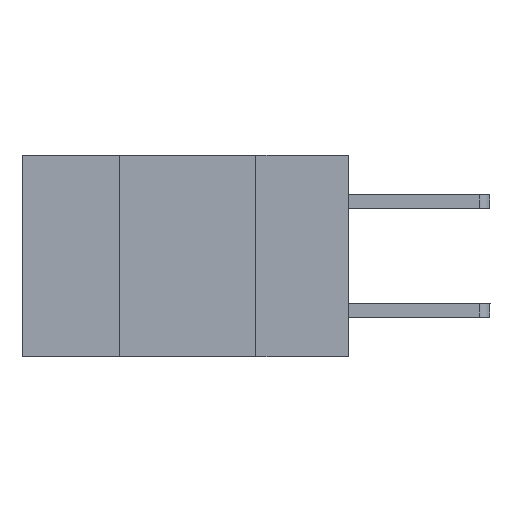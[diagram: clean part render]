
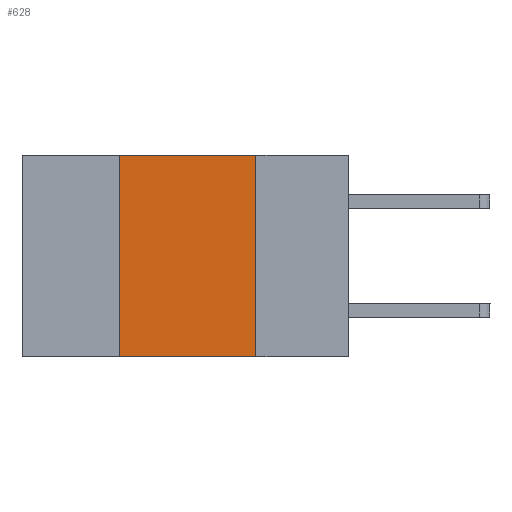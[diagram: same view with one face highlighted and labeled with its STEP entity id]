
A CAD part, left-side view. The second image highlights one B-rep face of the part: STEP entity #628.
In plain terms, the highlighted planar face has unit normal (-1, 0, 0).
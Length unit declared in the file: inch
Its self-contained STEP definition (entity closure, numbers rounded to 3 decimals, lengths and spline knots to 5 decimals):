
#43 = VECTOR ( 'NONE', #7409, 39.37008 ) ;
#469 = CARTESIAN_POINT ( 'NONE',  ( 0., 0.6, -0.37 ) ) ;
#628 = ADVANCED_FACE ( 'NONE', ( #2798 ), #4369, .F. ) ;
#1009 = CARTESIAN_POINT ( 'NONE',  ( 0., 0.17, 0. ) ) ;
#1123 = EDGE_CURVE ( 'NONE', #7954, #1808, #10056, .T. ) ;
#1143 = VECTOR ( 'NONE', #1589, 39.37008 ) ;
#1338 = LINE ( 'NONE', #1009, #43 ) ;
#1589 = DIRECTION ( 'NONE',  ( 0., 0., 1. ) ) ;
#1766 = EDGE_CURVE ( 'NONE', #7954, #2212, #9905, .T. ) ;
#1808 = VERTEX_POINT ( 'NONE', #9048 ) ;
#2044 = LINE ( 'NONE', #10238, #9132 ) ;
#2212 = VERTEX_POINT ( 'NONE', #3645 ) ;
#2516 = VERTEX_POINT ( 'NONE', #5108 ) ;
#2798 = FACE_OUTER_BOUND ( 'NONE', #9317, .T. ) ;
#2799 = DIRECTION ( 'NONE',  ( 1., 0., 0. ) ) ;
#3293 = ORIENTED_EDGE ( 'NONE', *, *, #1766, .F. ) ;
#3633 = DIRECTION ( 'NONE',  ( 0., -1., 0. ) ) ;
#3645 = CARTESIAN_POINT ( 'NONE',  ( 0., 0.42, 0. ) ) ;
#4081 = ORIENTED_EDGE ( 'NONE', *, *, #5012, .F. ) ;
#4369 = PLANE ( 'NONE',  #6369 ) ;
#5012 = EDGE_CURVE ( 'NONE', #2212, #2516, #2044, .T. ) ;
#5108 = CARTESIAN_POINT ( 'NONE',  ( 0., 0.17, 0. ) ) ;
#5318 = CARTESIAN_POINT ( 'NONE',  ( 0., 0.6, 0. ) ) ;
#5828 = ORIENTED_EDGE ( 'NONE', *, *, #8159, .F. ) ;
#5931 = ORIENTED_EDGE ( 'NONE', *, *, #1123, .T. ) ;
#6369 = AXIS2_PLACEMENT_3D ( 'NONE', #5318, #2799, #10193 ) ;
#6488 = CARTESIAN_POINT ( 'NONE',  ( 0., 0.42, 0. ) ) ;
#7409 = DIRECTION ( 'NONE',  ( 0., 0., -1. ) ) ;
#7812 = VECTOR ( 'NONE', #3633, 39.37008 ) ;
#7954 = VERTEX_POINT ( 'NONE', #10414 ) ;
#8159 = EDGE_CURVE ( 'NONE', #2516, #1808, #1338, .T. ) ;
#9048 = CARTESIAN_POINT ( 'NONE',  ( 0., 0.17, -0.37 ) ) ;
#9132 = VECTOR ( 'NONE', #9478, 39.37008 ) ;
#9317 = EDGE_LOOP ( 'NONE', ( #5828, #4081, #3293, #5931 ) ) ;
#9478 = DIRECTION ( 'NONE',  ( 0., -1., 0. ) ) ;
#9905 = LINE ( 'NONE', #6488, #1143 ) ;
#10056 = LINE ( 'NONE', #469, #7812 ) ;
#10193 = DIRECTION ( 'NONE',  ( 0., 0., -1. ) ) ;
#10238 = CARTESIAN_POINT ( 'NONE',  ( 0., 0.6, 0. ) ) ;
#10414 = CARTESIAN_POINT ( 'NONE',  ( 0., 0.42, -0.37 ) ) ;
